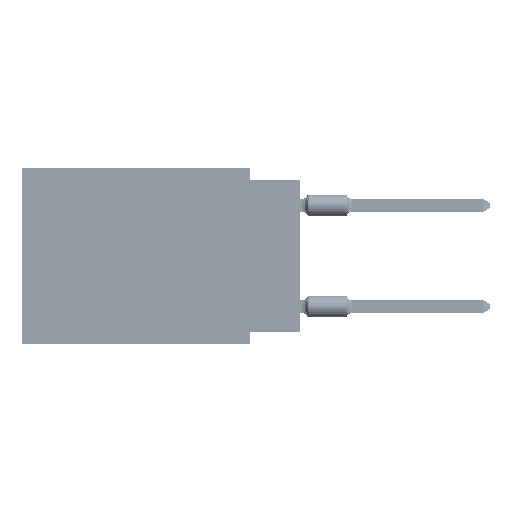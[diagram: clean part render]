
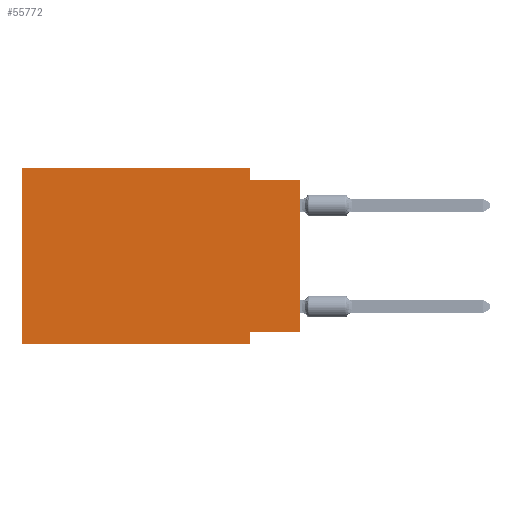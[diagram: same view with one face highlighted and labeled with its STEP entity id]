
A CAD part, left-side view. The second image highlights one B-rep face of the part: STEP entity #55772.
In plain terms, the highlighted planar face has unit normal (-1, 0, 0).
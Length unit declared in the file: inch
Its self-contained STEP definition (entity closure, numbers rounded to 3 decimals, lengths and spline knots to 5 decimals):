
#1229 = VECTOR ( 'NONE', #54113, 39.37008 ) ;
#3125 = EDGE_CURVE ( 'NONE', #39606, #103611, #65681, .T. ) ;
#5536 = ORIENTED_EDGE ( 'NONE', *, *, #43521, .F. ) ;
#5541 = LINE ( 'NONE', #15448, #57263 ) ;
#6518 = DIRECTION ( 'NONE',  ( 0., 0., -1. ) ) ;
#8443 = CARTESIAN_POINT ( 'NONE',  ( 0., 0.55, 0. ) ) ;
#10237 = CARTESIAN_POINT ( 'NONE',  ( 0., 0., -0.025 ) ) ;
#11685 = CARTESIAN_POINT ( 'NONE',  ( 0., 0.1, -0.025 ) ) ;
#14821 = CARTESIAN_POINT ( 'NONE',  ( 0., 0., -0.025 ) ) ;
#15448 = CARTESIAN_POINT ( 'NONE',  ( 0., 0.55, 0. ) ) ;
#15790 = DIRECTION ( 'NONE',  ( 0., -1., 0. ) ) ;
#16192 = DIRECTION ( 'NONE',  ( 1., 0., 0. ) ) ;
#17184 = DIRECTION ( 'NONE',  ( 0., 0., 1. ) ) ;
#17382 = VERTEX_POINT ( 'NONE', #14821 ) ;
#17987 = VECTOR ( 'NONE', #15790, 39.37008 ) ;
#18457 = LINE ( 'NONE', #10237, #1229 ) ;
#21786 = CARTESIAN_POINT ( 'NONE',  ( 0., 0., -0.325 ) ) ;
#24268 = DIRECTION ( 'NONE',  ( 0., 0., 1. ) ) ;
#27702 = CARTESIAN_POINT ( 'NONE',  ( 0., 0.1, -0.325 ) ) ;
#28116 = DIRECTION ( 'NONE',  ( 0., 1., 0. ) ) ;
#28709 = EDGE_CURVE ( 'NONE', #73605, #30354, #60219, .T. ) ;
#29473 = EDGE_CURVE ( 'NONE', #37358, #39606, #5541, .T. ) ;
#30354 = VERTEX_POINT ( 'NONE', #102308 ) ;
#31019 = ORIENTED_EDGE ( 'NONE', *, *, #3125, .F. ) ;
#33195 = CARTESIAN_POINT ( 'NONE',  ( 0., 0.55, 0. ) ) ;
#37358 = VERTEX_POINT ( 'NONE', #91091 ) ;
#39606 = VERTEX_POINT ( 'NONE', #44611 ) ;
#40650 = DIRECTION ( 'NONE',  ( 0., -1., 0. ) ) ;
#40909 = ORIENTED_EDGE ( 'NONE', *, *, #29473, .F. ) ;
#43521 = EDGE_CURVE ( 'NONE', #73605, #37358, #52882, .T. ) ;
#44136 = CARTESIAN_POINT ( 'NONE',  ( 0., 0., 0. ) ) ;
#44611 = CARTESIAN_POINT ( 'NONE',  ( 0., 0.1, 0. ) ) ;
#49338 = CARTESIAN_POINT ( 'NONE',  ( 0., 0.1, 0. ) ) ;
#52681 = LINE ( 'NONE', #88287, #100762 ) ;
#52882 = LINE ( 'NONE', #8443, #60938 ) ;
#53213 = ORIENTED_EDGE ( 'NONE', *, *, #53819, .F. ) ;
#53819 = EDGE_CURVE ( 'NONE', #57982, #80194, #73652, .T. ) ;
#54113 = DIRECTION ( 'NONE',  ( 0., -1., 0. ) ) ;
#55772 = ADVANCED_FACE ( 'NONE', ( #68238 ), #96255, .F. ) ;
#56178 = ORIENTED_EDGE ( 'NONE', *, *, #72516, .T. ) ;
#57263 = VECTOR ( 'NONE', #40650, 39.37008 ) ;
#57315 = EDGE_CURVE ( 'NONE', #103611, #17382, #18457, .T. ) ;
#57982 = VERTEX_POINT ( 'NONE', #21786 ) ;
#60219 = LINE ( 'NONE', #95854, #17987 ) ;
#60938 = VECTOR ( 'NONE', #24268, 39.37008 ) ;
#61821 = VECTOR ( 'NONE', #74445, 39.37008 ) ;
#61870 = EDGE_LOOP ( 'NONE', ( #56178, #97418, #31019, #40909, #5536, #78091, #79669, #53213 ) ) ;
#65681 = LINE ( 'NONE', #49338, #61821 ) ;
#68238 = FACE_OUTER_BOUND ( 'NONE', #61870, .T. ) ;
#70072 = AXIS2_PLACEMENT_3D ( 'NONE', #33195, #16192, #113227 ) ;
#70957 = LINE ( 'NONE', #44136, #111509 ) ;
#72516 = EDGE_CURVE ( 'NONE', #57982, #17382, #70957, .T. ) ;
#73605 = VERTEX_POINT ( 'NONE', #73656 ) ;
#73652 = LINE ( 'NONE', #81815, #94278 ) ;
#73656 = CARTESIAN_POINT ( 'NONE',  ( 0., 0.55, -0.35 ) ) ;
#74445 = DIRECTION ( 'NONE',  ( 0., 0., -1. ) ) ;
#78091 = ORIENTED_EDGE ( 'NONE', *, *, #28709, .T. ) ;
#79669 = ORIENTED_EDGE ( 'NONE', *, *, #103396, .F. ) ;
#80194 = VERTEX_POINT ( 'NONE', #27702 ) ;
#81815 = CARTESIAN_POINT ( 'NONE',  ( 0., 0., -0.325 ) ) ;
#88287 = CARTESIAN_POINT ( 'NONE',  ( 0., 0.1, -0.35 ) ) ;
#91091 = CARTESIAN_POINT ( 'NONE',  ( 0., 0.55, 0. ) ) ;
#94278 = VECTOR ( 'NONE', #28116, 39.37008 ) ;
#95854 = CARTESIAN_POINT ( 'NONE',  ( 0., 0.55, -0.35 ) ) ;
#96255 = PLANE ( 'NONE',  #70072 ) ;
#97418 = ORIENTED_EDGE ( 'NONE', *, *, #57315, .F. ) ;
#100762 = VECTOR ( 'NONE', #6518, 39.37008 ) ;
#102308 = CARTESIAN_POINT ( 'NONE',  ( 0., 0.1, -0.35 ) ) ;
#103396 = EDGE_CURVE ( 'NONE', #80194, #30354, #52681, .T. ) ;
#103611 = VERTEX_POINT ( 'NONE', #11685 ) ;
#111509 = VECTOR ( 'NONE', #17184, 39.37008 ) ;
#113227 = DIRECTION ( 'NONE',  ( 0., 0., -1. ) ) ;
